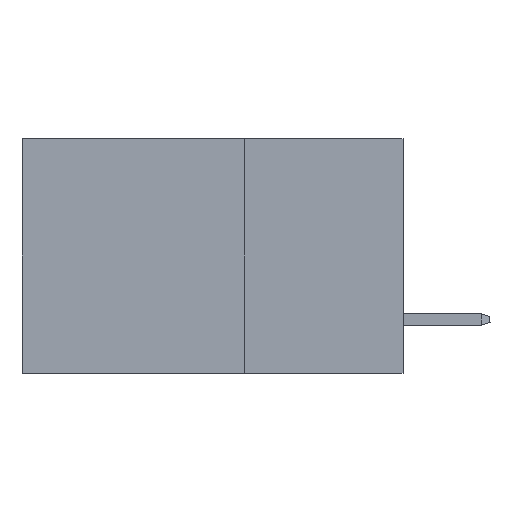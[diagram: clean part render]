
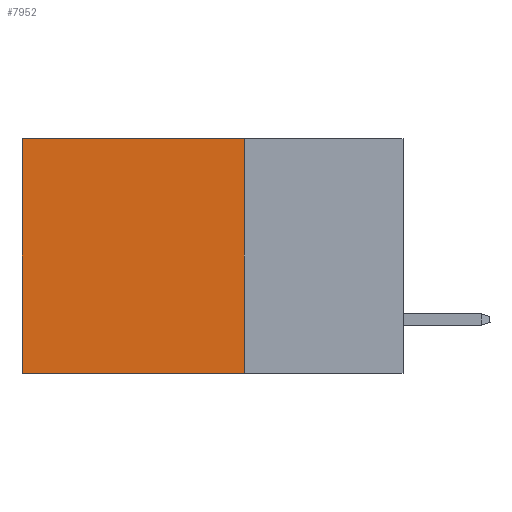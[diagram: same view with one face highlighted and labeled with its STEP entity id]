
A CAD part, left-side view. The second image highlights one B-rep face of the part: STEP entity #7952.
In plain terms, the highlighted planar face has unit normal (-1, 0, 0).
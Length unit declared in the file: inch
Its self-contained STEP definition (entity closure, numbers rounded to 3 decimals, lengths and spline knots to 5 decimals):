
#491 = EDGE_LOOP ( 'NONE', ( #5686, #1527, #1429, #24473 ) ) ;
#612 = EDGE_CURVE ( 'NONE', #857, #11250, #17164, .T. ) ;
#857 = VERTEX_POINT ( 'NONE', #10289 ) ;
#1429 = ORIENTED_EDGE ( 'NONE', *, *, #5688, .F. ) ;
#1527 = ORIENTED_EDGE ( 'NONE', *, *, #15968, .F. ) ;
#1843 = FACE_OUTER_BOUND ( 'NONE', #491, .T. ) ;
#2075 = EDGE_CURVE ( 'NONE', #11250, #25357, #22062, .T. ) ;
#3630 = CARTESIAN_POINT ( 'NONE',  ( 0.2875, 0.25, -0.37 ) ) ;
#4696 = VECTOR ( 'NONE', #8126, 39.37008 ) ;
#5686 = ORIENTED_EDGE ( 'NONE', *, *, #2075, .T. ) ;
#5688 = EDGE_CURVE ( 'NONE', #857, #25799, #11953, .T. ) ;
#5981 = CARTESIAN_POINT ( 'NONE',  ( 0.2875, 0.25, 0. ) ) ;
#7114 = VECTOR ( 'NONE', #17304, 39.37008 ) ;
#7801 = DIRECTION ( 'NONE',  ( 1., 0., 0. ) ) ;
#7952 = ADVANCED_FACE ( 'NONE', ( #1843 ), #26053, .F. ) ;
#8126 = DIRECTION ( 'NONE',  ( 0., 0., -1. ) ) ;
#8817 = VECTOR ( 'NONE', #19504, 39.37008 ) ;
#9888 = AXIS2_PLACEMENT_3D ( 'NONE', #17982, #7801, #14011 ) ;
#10289 = CARTESIAN_POINT ( 'NONE',  ( 0.2875, 0.25, 0. ) ) ;
#11227 = CARTESIAN_POINT ( 'NONE',  ( 0.2875, 0.25, 0. ) ) ;
#11250 = VERTEX_POINT ( 'NONE', #25011 ) ;
#11268 = CARTESIAN_POINT ( 'NONE',  ( 0.2875, 0.6, 0. ) ) ;
#11953 = LINE ( 'NONE', #5981, #4696 ) ;
#13290 = LINE ( 'NONE', #19383, #8817 ) ;
#14011 = DIRECTION ( 'NONE',  ( 0., 0., -1. ) ) ;
#15968 = EDGE_CURVE ( 'NONE', #25799, #25357, #13290, .T. ) ;
#17164 = LINE ( 'NONE', #11227, #7114 ) ;
#17304 = DIRECTION ( 'NONE',  ( 0., 1., 0. ) ) ;
#17570 = VECTOR ( 'NONE', #23412, 39.37008 ) ;
#17982 = CARTESIAN_POINT ( 'NONE',  ( 0.2875, 0.25, 0. ) ) ;
#19383 = CARTESIAN_POINT ( 'NONE',  ( 0.2875, 0.25, -0.37 ) ) ;
#19504 = DIRECTION ( 'NONE',  ( 0., 1., 0. ) ) ;
#22062 = LINE ( 'NONE', #11268, #17570 ) ;
#23412 = DIRECTION ( 'NONE',  ( 0., 0., -1. ) ) ;
#24473 = ORIENTED_EDGE ( 'NONE', *, *, #612, .T. ) ;
#25011 = CARTESIAN_POINT ( 'NONE',  ( 0.2875, 0.6, 0. ) ) ;
#25357 = VERTEX_POINT ( 'NONE', #26028 ) ;
#25799 = VERTEX_POINT ( 'NONE', #3630 ) ;
#26028 = CARTESIAN_POINT ( 'NONE',  ( 0.2875, 0.6, -0.37 ) ) ;
#26053 = PLANE ( 'NONE',  #9888 ) ;
